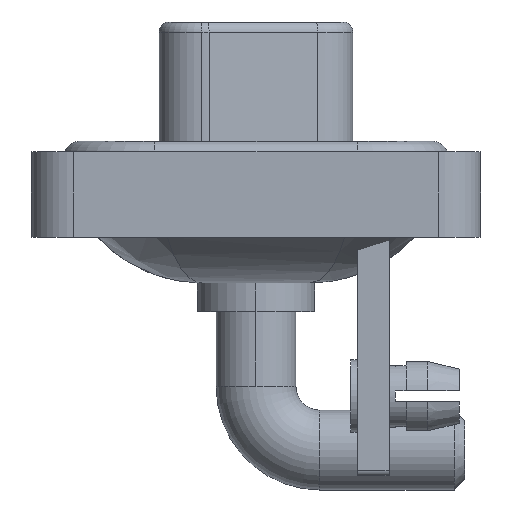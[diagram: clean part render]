
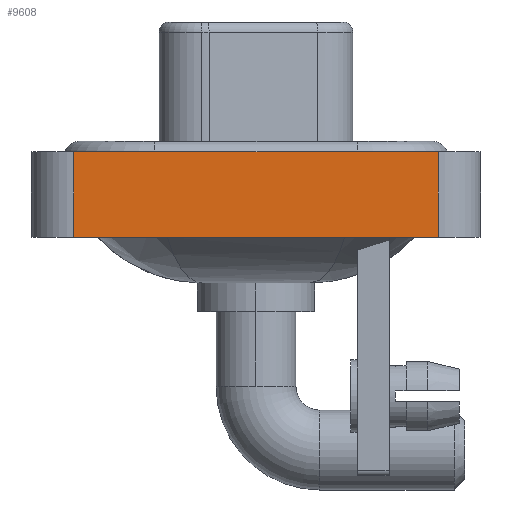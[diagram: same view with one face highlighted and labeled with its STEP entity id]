
A CAD part, left-side view. The second image highlights one B-rep face of the part: STEP entity #9608.
In plain terms, the highlighted planar face has unit normal (-1, 0, 0).
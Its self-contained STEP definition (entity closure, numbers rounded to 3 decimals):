
#1011 = ORIENTED_EDGE ( 'NONE', *, *, #7363, .T. ) ;
#2665 = CARTESIAN_POINT ( 'NONE',  ( -7.25, -8.55, -3.6 ) ) ;
#2745 = DIRECTION ( 'NONE',  ( 0., 0., 1. ) ) ;
#3106 = VERTEX_POINT ( 'NONE', #17120 ) ;
#3808 = LINE ( 'NONE', #9193, #16731 ) ;
#4183 = DIRECTION ( 'NONE',  ( 0., -1., 0. ) ) ;
#4299 = DIRECTION ( 'NONE',  ( 0., -1., 0. ) ) ;
#4325 = ORIENTED_EDGE ( 'NONE', *, *, #13072, .T. ) ;
#4545 = CARTESIAN_POINT ( 'NONE',  ( -7.25, -8.55, -3.6 ) ) ;
#4557 = VERTEX_POINT ( 'NONE', #2665 ) ;
#4834 = CARTESIAN_POINT ( 'NONE',  ( -7.25, 8.55, -3.6 ) ) ;
#5413 = CARTESIAN_POINT ( 'NONE',  ( -7.25, -8.55, -3.6 ) ) ;
#5496 = PLANE ( 'NONE',  #13398 ) ;
#5583 = VECTOR ( 'NONE', #4299, 1000. ) ;
#6241 = EDGE_CURVE ( 'NONE', #16031, #13996, #7829, .T. ) ;
#6556 = ORIENTED_EDGE ( 'NONE', *, *, #15480, .F. ) ;
#6716 = DIRECTION ( 'NONE',  ( 0., 0., 1. ) ) ;
#7063 = CARTESIAN_POINT ( 'NONE',  ( -7.25, 8.55, 0.4 ) ) ;
#7363 = EDGE_CURVE ( 'NONE', #4557, #3106, #3808, .T. ) ;
#7829 = LINE ( 'NONE', #4834, #14169 ) ;
#8200 = ORIENTED_EDGE ( 'NONE', *, *, #6241, .F. ) ;
#8507 = EDGE_LOOP ( 'NONE', ( #1011, #6556, #8200, #4325 ) ) ;
#8963 = FACE_OUTER_BOUND ( 'NONE', #8507, .T. ) ;
#9193 = CARTESIAN_POINT ( 'NONE',  ( -7.25, -8.55, -3.6 ) ) ;
#9608 = ADVANCED_FACE ( 'NONE', ( #8963 ), #5496, .T. ) ;
#12586 = LINE ( 'NONE', #4545, #17177 ) ;
#13072 = EDGE_CURVE ( 'NONE', #16031, #4557, #12586, .T. ) ;
#13398 = AXIS2_PLACEMENT_3D ( 'NONE', #5413, #13535, #2745 ) ;
#13535 = DIRECTION ( 'NONE',  ( -1., 0., 0. ) ) ;
#13996 = VERTEX_POINT ( 'NONE', #7063 ) ;
#14169 = VECTOR ( 'NONE', #14295, 1000. ) ;
#14295 = DIRECTION ( 'NONE',  ( 0., 0., 1. ) ) ;
#15176 = CARTESIAN_POINT ( 'NONE',  ( -7.25, -8.55, 0.4 ) ) ;
#15480 = EDGE_CURVE ( 'NONE', #13996, #3106, #16152, .T. ) ;
#16031 = VERTEX_POINT ( 'NONE', #17457 ) ;
#16152 = LINE ( 'NONE', #15176, #5583 ) ;
#16731 = VECTOR ( 'NONE', #6716, 1000. ) ;
#17120 = CARTESIAN_POINT ( 'NONE',  ( -7.25, -8.55, 0.4 ) ) ;
#17177 = VECTOR ( 'NONE', #4183, 1000. ) ;
#17457 = CARTESIAN_POINT ( 'NONE',  ( -7.25, 8.55, -3.6 ) ) ;
